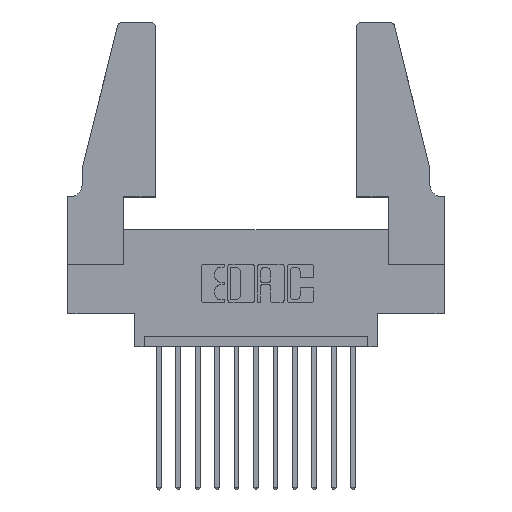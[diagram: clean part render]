
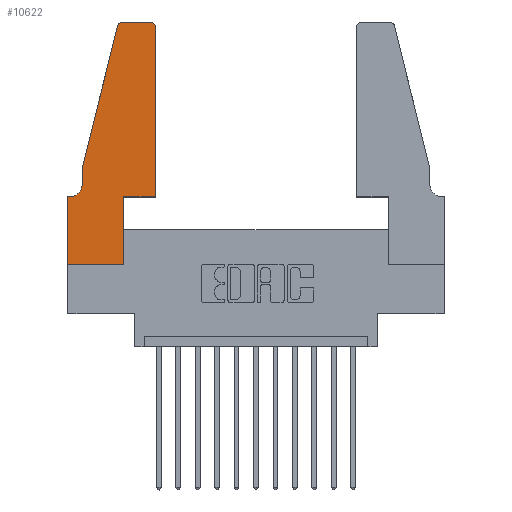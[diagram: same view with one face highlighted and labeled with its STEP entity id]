
A CAD part, top view. The second image highlights one B-rep face of the part: STEP entity #10622.
In plain terms, the highlighted planar face has unit normal (0, 0, 1).
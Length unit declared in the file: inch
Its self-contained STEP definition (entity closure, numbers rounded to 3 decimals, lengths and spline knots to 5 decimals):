
#8 = AXIS2_PLACEMENT_3D ( 'NONE', #11608, #4802, #7226 ) ;
#34 = VECTOR ( 'NONE', #10446, 39.37008 ) ;
#447 = DIRECTION ( 'NONE',  ( 0., 1., 0. ) ) ;
#591 = EDGE_CURVE ( 'NONE', #12891, #14025, #3811, .T. ) ;
#621 = LINE ( 'NONE', #7861, #3832 ) ;
#779 = DIRECTION ( 'NONE',  ( 1., 0., 0. ) ) ;
#825 = DIRECTION ( 'NONE',  ( -1., 0., 0. ) ) ;
#1025 = AXIS2_PLACEMENT_3D ( 'NONE', #5343, #3032, #825 ) ;
#1489 = CARTESIAN_POINT ( 'NONE',  ( 0.0755, 0.5, 0.37 ) ) ;
#1540 = EDGE_CURVE ( 'NONE', #11805, #6155, #7682, .T. ) ;
#1729 = VECTOR ( 'NONE', #14024, 39.37008 ) ;
#1919 = CARTESIAN_POINT ( 'NONE',  ( 0., 0., 0.37 ) ) ;
#1982 = VERTEX_POINT ( 'NONE', #10018 ) ;
#2086 = ORIENTED_EDGE ( 'NONE', *, *, #12525, .T. ) ;
#2366 = FACE_OUTER_BOUND ( 'NONE', #11722, .T. ) ;
#2783 = CIRCLE ( 'NONE', #8, 0.03 ) ;
#3032 = DIRECTION ( 'NONE',  ( 0., 0., -1. ) ) ;
#3107 = CARTESIAN_POINT ( 'NONE',  ( 0.4505, 0.35, 0.37 ) ) ;
#3108 = LINE ( 'NONE', #5817, #34 ) ;
#3317 = EDGE_CURVE ( 'NONE', #9926, #9612, #7100, .T. ) ;
#3353 = ORIENTED_EDGE ( 'NONE', *, *, #13069, .T. ) ;
#3459 = VECTOR ( 'NONE', #4514, 39.37008 ) ;
#3650 = EDGE_CURVE ( 'NONE', #1982, #11129, #9766, .T. ) ;
#3695 = ORIENTED_EDGE ( 'NONE', *, *, #5725, .T. ) ;
#3811 = LINE ( 'NONE', #7835, #3459 ) ;
#3832 = VECTOR ( 'NONE', #11223, 39.37008 ) ;
#4035 = CARTESIAN_POINT ( 'NONE',  ( 0.0755, 0.35, 0.37 ) ) ;
#4298 = CARTESIAN_POINT ( 'NONE',  ( 0.4205, 1.25, 0.37 ) ) ;
#4394 = CARTESIAN_POINT ( 'NONE',  ( 0.0755, 0.5, 0.37 ) ) ;
#4409 = ORIENTED_EDGE ( 'NONE', *, *, #9528, .T. ) ;
#4417 = ORIENTED_EDGE ( 'NONE', *, *, #3317, .T. ) ;
#4514 = DIRECTION ( 'NONE',  ( 0., 1., 0. ) ) ;
#4529 = VERTEX_POINT ( 'NONE', #1919 ) ;
#4729 = VERTEX_POINT ( 'NONE', #6381 ) ;
#4802 = DIRECTION ( 'NONE',  ( 0., 0., 1. ) ) ;
#4858 = CARTESIAN_POINT ( 'NONE',  ( 0.4505, 0.35, 0.37 ) ) ;
#4918 = AXIS2_PLACEMENT_3D ( 'NONE', #6135, #14086, #5025 ) ;
#5025 = DIRECTION ( 'NONE',  ( 1., 0., 0. ) ) ;
#5065 = VECTOR ( 'NONE', #13643, 39.37008 ) ;
#5343 = CARTESIAN_POINT ( 'NONE',  ( 0.0055, 0.42, 0.37 ) ) ;
#5515 = LINE ( 'NONE', #8921, #10867 ) ;
#5725 = EDGE_CURVE ( 'NONE', #11129, #13411, #9005, .T. ) ;
#5808 = CARTESIAN_POINT ( 'NONE',  ( 0.4505, 1.22, 0.37 ) ) ;
#5817 = CARTESIAN_POINT ( 'NONE',  ( 0., 0., 0.37 ) ) ;
#6135 = CARTESIAN_POINT ( 'NONE',  ( 0.284, 1.22, 0.37 ) ) ;
#6155 = VERTEX_POINT ( 'NONE', #5808 ) ;
#6381 = CARTESIAN_POINT ( 'NONE',  ( 0.0755, 0.5, 0.37 ) ) ;
#6699 = ORIENTED_EDGE ( 'NONE', *, *, #10257, .T. ) ;
#6800 = CARTESIAN_POINT ( 'NONE',  ( 0.2865, 0., 0.37 ) ) ;
#6878 = CARTESIAN_POINT ( 'NONE',  ( 0.25487, 1.22718, 0.37 ) ) ;
#7021 = LINE ( 'NONE', #4394, #5065 ) ;
#7100 = CIRCLE ( 'NONE', #4918, 0.03 ) ;
#7152 = VERTEX_POINT ( 'NONE', #4298 ) ;
#7164 = EDGE_CURVE ( 'NONE', #13411, #4529, #5515, .T. ) ;
#7226 = DIRECTION ( 'NONE',  ( 1., 0., 0. ) ) ;
#7682 = LINE ( 'NONE', #12724, #14463 ) ;
#7762 = CARTESIAN_POINT ( 'NONE',  ( 0., 0.35, 0.37 ) ) ;
#7835 = CARTESIAN_POINT ( 'NONE',  ( 0.2865, 0.35, 0.37 ) ) ;
#7861 = CARTESIAN_POINT ( 'NONE',  ( 0.2605, 1.25, 0.37 ) ) ;
#7939 = VECTOR ( 'NONE', #11622, 39.37008 ) ;
#8467 = ORIENTED_EDGE ( 'NONE', *, *, #591, .T. ) ;
#8491 = LINE ( 'NONE', #1489, #1729 ) ;
#8848 = VECTOR ( 'NONE', #12065, 39.37008 ) ;
#8921 = CARTESIAN_POINT ( 'NONE',  ( 0., 0., 0.37 ) ) ;
#9005 = LINE ( 'NONE', #4035, #8848 ) ;
#9528 = EDGE_CURVE ( 'NONE', #4729, #1982, #7021, .T. ) ;
#9612 = VERTEX_POINT ( 'NONE', #6878 ) ;
#9686 = PLANE ( 'NONE',  #10691 ) ;
#9759 = CARTESIAN_POINT ( 'NONE',  ( 0.284, 1.25, 0.37 ) ) ;
#9766 = CIRCLE ( 'NONE', #1025, 0.07 ) ;
#9926 = VERTEX_POINT ( 'NONE', #9759 ) ;
#10018 = CARTESIAN_POINT ( 'NONE',  ( 0.0755, 0.42, 0.37 ) ) ;
#10022 = DIRECTION ( 'NONE',  ( 0., -1., 0. ) ) ;
#10144 = ORIENTED_EDGE ( 'NONE', *, *, #7164, .T. ) ;
#10257 = EDGE_CURVE ( 'NONE', #4529, #12891, #3108, .T. ) ;
#10446 = DIRECTION ( 'NONE',  ( 1., 0., 0. ) ) ;
#10622 = ADVANCED_FACE ( 'NONE', ( #2366 ), #9686, .T. ) ;
#10691 = AXIS2_PLACEMENT_3D ( 'NONE', #14408, #10842, #779 ) ;
#10750 = ORIENTED_EDGE ( 'NONE', *, *, #12404, .T. ) ;
#10798 = ORIENTED_EDGE ( 'NONE', *, *, #1540, .T. ) ;
#10842 = DIRECTION ( 'NONE',  ( 0., 0., 1. ) ) ;
#10867 = VECTOR ( 'NONE', #10022, 39.37008 ) ;
#11129 = VERTEX_POINT ( 'NONE', #14154 ) ;
#11223 = DIRECTION ( 'NONE',  ( -1., 0., 0. ) ) ;
#11608 = CARTESIAN_POINT ( 'NONE',  ( 0.4205, 1.22, 0.37 ) ) ;
#11622 = DIRECTION ( 'NONE',  ( 1., 0., 0. ) ) ;
#11722 = EDGE_LOOP ( 'NONE', ( #11997, #4417, #2086, #4409, #12776, #3695, #10144, #6699, #8467, #10750, #10798, #3353 ) ) ;
#11805 = VERTEX_POINT ( 'NONE', #3107 ) ;
#11997 = ORIENTED_EDGE ( 'NONE', *, *, #13480, .T. ) ;
#12065 = DIRECTION ( 'NONE',  ( -1., 0., 0. ) ) ;
#12404 = EDGE_CURVE ( 'NONE', #14025, #11805, #14198, .T. ) ;
#12525 = EDGE_CURVE ( 'NONE', #9612, #4729, #8491, .T. ) ;
#12724 = CARTESIAN_POINT ( 'NONE',  ( 0.4505, 0.35, 0.37 ) ) ;
#12776 = ORIENTED_EDGE ( 'NONE', *, *, #3650, .T. ) ;
#12891 = VERTEX_POINT ( 'NONE', #6800 ) ;
#13069 = EDGE_CURVE ( 'NONE', #6155, #7152, #2783, .T. ) ;
#13411 = VERTEX_POINT ( 'NONE', #7762 ) ;
#13480 = EDGE_CURVE ( 'NONE', #7152, #9926, #621, .T. ) ;
#13643 = DIRECTION ( 'NONE',  ( 0., -1., 0. ) ) ;
#14024 = DIRECTION ( 'NONE',  ( -0.239, -0.971, 0. ) ) ;
#14025 = VERTEX_POINT ( 'NONE', #14644 ) ;
#14086 = DIRECTION ( 'NONE',  ( 0., 0., 1. ) ) ;
#14154 = CARTESIAN_POINT ( 'NONE',  ( 0.0055, 0.35, 0.37 ) ) ;
#14198 = LINE ( 'NONE', #4858, #7939 ) ;
#14408 = CARTESIAN_POINT ( 'NONE',  ( 0., 0.35, 0.37 ) ) ;
#14463 = VECTOR ( 'NONE', #447, 39.37008 ) ;
#14644 = CARTESIAN_POINT ( 'NONE',  ( 0.2865, 0.35, 0.37 ) ) ;
